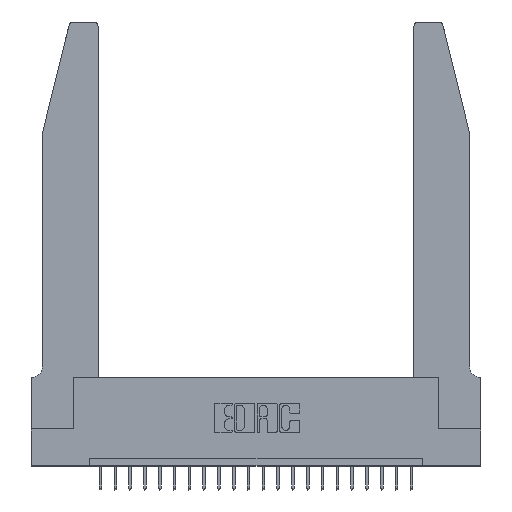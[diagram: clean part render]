
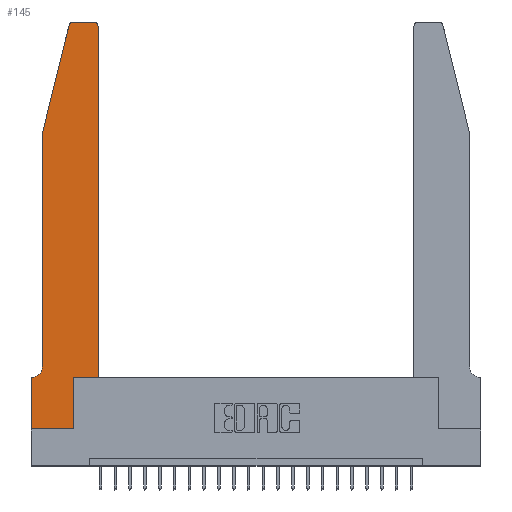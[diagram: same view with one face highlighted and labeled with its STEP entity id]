
A CAD part, top view. The second image highlights one B-rep face of the part: STEP entity #145.
In plain terms, the highlighted planar face has unit normal (0, 0, 1).
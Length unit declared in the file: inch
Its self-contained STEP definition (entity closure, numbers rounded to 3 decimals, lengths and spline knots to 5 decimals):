
#145 = ADVANCED_FACE ( 'NONE', ( #2668 ), #13463, .T. ) ;
#551 = DIRECTION ( 'NONE',  ( 0., -1., 0. ) ) ;
#575 = EDGE_CURVE ( 'NONE', #2136, #5407, #19499, .T. ) ;
#1301 = DIRECTION ( 'NONE',  ( 1., 0., 0. ) ) ;
#1424 = VECTOR ( 'NONE', #13688, 39.37008 ) ;
#1883 = DIRECTION ( 'NONE',  ( 0., 1., 0. ) ) ;
#2056 = CARTESIAN_POINT ( 'NONE',  ( 0.284, 2.75, 0.37 ) ) ;
#2136 = VERTEX_POINT ( 'NONE', #6323 ) ;
#2148 = ORIENTED_EDGE ( 'NONE', *, *, #22743, .T. ) ;
#2325 = CIRCLE ( 'NONE', #3177, 0.07 ) ;
#2668 = FACE_OUTER_BOUND ( 'NONE', #13771, .T. ) ;
#2942 = DIRECTION ( 'NONE',  ( 0., 0., 1. ) ) ;
#3110 = CARTESIAN_POINT ( 'NONE',  ( 0.2865, 0., 0.37 ) ) ;
#3161 = CARTESIAN_POINT ( 'NONE',  ( 0.4505, 2.72, 0.37 ) ) ;
#3177 = AXIS2_PLACEMENT_3D ( 'NONE', #8177, #21317, #14826 ) ;
#3381 = CARTESIAN_POINT ( 'NONE',  ( 0.4205, 2.72, 0.37 ) ) ;
#3481 = EDGE_CURVE ( 'NONE', #17620, #5835, #21562, .T. ) ;
#3629 = CARTESIAN_POINT ( 'NONE',  ( 0.0755, 0.35, 0.37 ) ) ;
#4424 = VECTOR ( 'NONE', #1301, 39.37008 ) ;
#4488 = DIRECTION ( 'NONE',  ( -1., 0., 0. ) ) ;
#4725 = CARTESIAN_POINT ( 'NONE',  ( 0.0055, 0.35, 0.37 ) ) ;
#4775 = EDGE_CURVE ( 'NONE', #14106, #16845, #5838, .T. ) ;
#5004 = LINE ( 'NONE', #19259, #18382 ) ;
#5039 = EDGE_CURVE ( 'NONE', #21031, #19540, #22933, .T. ) ;
#5407 = VERTEX_POINT ( 'NONE', #14299 ) ;
#5556 = ORIENTED_EDGE ( 'NONE', *, *, #3481, .T. ) ;
#5835 = VERTEX_POINT ( 'NONE', #3161 ) ;
#5838 = LINE ( 'NONE', #9200, #18903 ) ;
#6064 = DIRECTION ( 'NONE',  ( 0., 0., 1. ) ) ;
#6178 = ORIENTED_EDGE ( 'NONE', *, *, #14192, .T. ) ;
#6323 = CARTESIAN_POINT ( 'NONE',  ( 0., 0.35, 0.37 ) ) ;
#6383 = CARTESIAN_POINT ( 'NONE',  ( 0.4505, 0.35, 0.37 ) ) ;
#7155 = DIRECTION ( 'NONE',  ( 0., 0., 1. ) ) ;
#7460 = DIRECTION ( 'NONE',  ( -1., 0., 0. ) ) ;
#7576 = VERTEX_POINT ( 'NONE', #4725 ) ;
#7970 = CARTESIAN_POINT ( 'NONE',  ( 0.0755, 2., 0.37 ) ) ;
#7986 = ORIENTED_EDGE ( 'NONE', *, *, #14527, .T. ) ;
#8012 = ORIENTED_EDGE ( 'NONE', *, *, #8998, .T. ) ;
#8161 = VECTOR ( 'NONE', #15375, 39.37008 ) ;
#8177 = CARTESIAN_POINT ( 'NONE',  ( 0.0055, 0.42, 0.37 ) ) ;
#8475 = DIRECTION ( 'NONE',  ( 1., 0., 0. ) ) ;
#8774 = CARTESIAN_POINT ( 'NONE',  ( 0., 0., 0.37 ) ) ;
#8990 = DIRECTION ( 'NONE',  ( 1., 0., 0. ) ) ;
#8998 = EDGE_CURVE ( 'NONE', #19971, #19452, #5004, .T. ) ;
#9109 = EDGE_CURVE ( 'NONE', #5407, #14106, #17817, .T. ) ;
#9200 = CARTESIAN_POINT ( 'NONE',  ( 0.2865, 0.35, 0.37 ) ) ;
#10800 = ORIENTED_EDGE ( 'NONE', *, *, #16372, .T. ) ;
#11315 = EDGE_CURVE ( 'NONE', #7576, #2136, #21323, .T. ) ;
#11371 = CARTESIAN_POINT ( 'NONE',  ( 0.4505, 0.35, 0.37 ) ) ;
#11444 = ORIENTED_EDGE ( 'NONE', *, *, #11315, .T. ) ;
#11597 = DIRECTION ( 'NONE',  ( 0., -1., 0. ) ) ;
#11639 = AXIS2_PLACEMENT_3D ( 'NONE', #3381, #7155, #8990 ) ;
#11795 = CARTESIAN_POINT ( 'NONE',  ( 0.0755, 0.42, 0.37 ) ) ;
#12470 = CARTESIAN_POINT ( 'NONE',  ( 0., 0., 0.37 ) ) ;
#13012 = ORIENTED_EDGE ( 'NONE', *, *, #4775, .T. ) ;
#13339 = CIRCLE ( 'NONE', #11639, 0.03 ) ;
#13343 = ORIENTED_EDGE ( 'NONE', *, *, #15622, .T. ) ;
#13354 = AXIS2_PLACEMENT_3D ( 'NONE', #19598, #2942, #8475 ) ;
#13463 = PLANE ( 'NONE',  #17558 ) ;
#13534 = ORIENTED_EDGE ( 'NONE', *, *, #5039, .T. ) ;
#13688 = DIRECTION ( 'NONE',  ( 1., 0., 0. ) ) ;
#13771 = EDGE_LOOP ( 'NONE', ( #8012, #10800, #2148, #13534, #6178, #11444, #18439, #15842, #13012, #7986, #5556, #13343 ) ) ;
#14106 = VERTEX_POINT ( 'NONE', #3110 ) ;
#14192 = EDGE_CURVE ( 'NONE', #19540, #7576, #2325, .T. ) ;
#14299 = CARTESIAN_POINT ( 'NONE',  ( 0., 0., 0.37 ) ) ;
#14527 = EDGE_CURVE ( 'NONE', #16845, #17620, #23807, .T. ) ;
#14826 = DIRECTION ( 'NONE',  ( -1., 0., 0. ) ) ;
#15020 = CARTESIAN_POINT ( 'NONE',  ( 0.4205, 2.75, 0.37 ) ) ;
#15375 = DIRECTION ( 'NONE',  ( -0.239, -0.971, 0. ) ) ;
#15622 = EDGE_CURVE ( 'NONE', #5835, #19971, #13339, .T. ) ;
#15842 = ORIENTED_EDGE ( 'NONE', *, *, #9109, .T. ) ;
#16098 = CARTESIAN_POINT ( 'NONE',  ( 0.25487, 2.72718, 0.37 ) ) ;
#16372 = EDGE_CURVE ( 'NONE', #19452, #22104, #20831, .T. ) ;
#16845 = VERTEX_POINT ( 'NONE', #19222 ) ;
#17194 = CARTESIAN_POINT ( 'NONE',  ( 0., 0.35, 0.37 ) ) ;
#17225 = VECTOR ( 'NONE', #11597, 39.37008 ) ;
#17558 = AXIS2_PLACEMENT_3D ( 'NONE', #17194, #6064, #19046 ) ;
#17620 = VERTEX_POINT ( 'NONE', #23879 ) ;
#17633 = CARTESIAN_POINT ( 'NONE',  ( 0.0755, 2., 0.37 ) ) ;
#17817 = LINE ( 'NONE', #12470, #4424 ) ;
#18382 = VECTOR ( 'NONE', #4488, 39.37008 ) ;
#18439 = ORIENTED_EDGE ( 'NONE', *, *, #575, .T. ) ;
#18672 = VECTOR ( 'NONE', #20680, 39.37008 ) ;
#18903 = VECTOR ( 'NONE', #1883, 39.37008 ) ;
#19046 = DIRECTION ( 'NONE',  ( 1., 0., 0. ) ) ;
#19222 = CARTESIAN_POINT ( 'NONE',  ( 0.2865, 0.35, 0.37 ) ) ;
#19259 = CARTESIAN_POINT ( 'NONE',  ( 0.2605, 2.75, 0.37 ) ) ;
#19452 = VERTEX_POINT ( 'NONE', #2056 ) ;
#19499 = LINE ( 'NONE', #8774, #17225 ) ;
#19540 = VERTEX_POINT ( 'NONE', #11795 ) ;
#19598 = CARTESIAN_POINT ( 'NONE',  ( 0.284, 2.72, 0.37 ) ) ;
#19971 = VERTEX_POINT ( 'NONE', #15020 ) ;
#20361 = LINE ( 'NONE', #7970, #8161 ) ;
#20680 = DIRECTION ( 'NONE',  ( 0., 1., 0. ) ) ;
#20831 = CIRCLE ( 'NONE', #13354, 0.03 ) ;
#20911 = VECTOR ( 'NONE', #551, 39.37008 ) ;
#21031 = VERTEX_POINT ( 'NONE', #21893 ) ;
#21317 = DIRECTION ( 'NONE',  ( 0., 0., -1. ) ) ;
#21323 = LINE ( 'NONE', #3629, #21920 ) ;
#21562 = LINE ( 'NONE', #11371, #18672 ) ;
#21893 = CARTESIAN_POINT ( 'NONE',  ( 0.0755, 2., 0.37 ) ) ;
#21920 = VECTOR ( 'NONE', #7460, 39.37008 ) ;
#22104 = VERTEX_POINT ( 'NONE', #16098 ) ;
#22743 = EDGE_CURVE ( 'NONE', #22104, #21031, #20361, .T. ) ;
#22933 = LINE ( 'NONE', #17633, #20911 ) ;
#23807 = LINE ( 'NONE', #6383, #1424 ) ;
#23879 = CARTESIAN_POINT ( 'NONE',  ( 0.4505, 0.35, 0.37 ) ) ;
